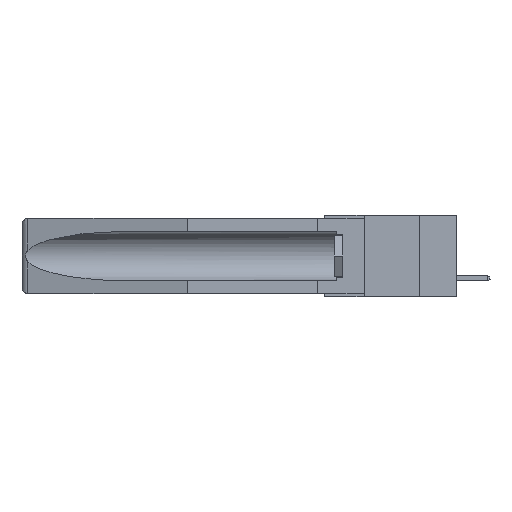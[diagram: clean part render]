
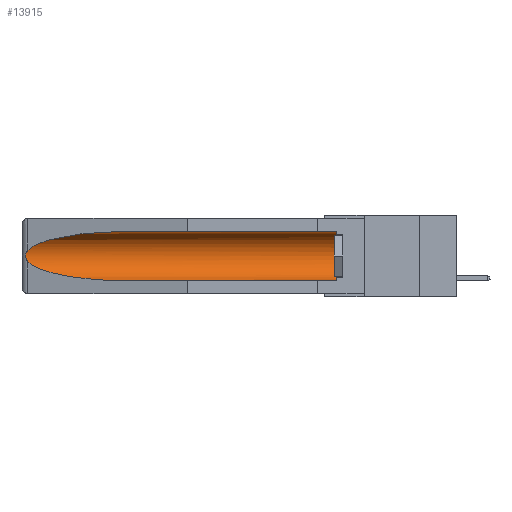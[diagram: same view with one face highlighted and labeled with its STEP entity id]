
A CAD part, left-side view. The second image highlights one B-rep face of the part: STEP entity #13915.
In plain terms, the highlighted cylindrical face has radius 2.857 mm (diameter 5.715 mm), a partial arc.
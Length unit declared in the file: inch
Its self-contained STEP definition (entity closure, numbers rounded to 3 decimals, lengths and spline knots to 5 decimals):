
#265 = EDGE_CURVE ( 'NONE', #20814, #21322, #21189, .T. ) ;
#880 = VERTEX_POINT ( 'NONE', #18249 ) ;
#1745 = CARTESIAN_POINT ( 'NONE',  ( 0.155, 0.126, -0.059 ) ) ;
#2369 = EDGE_CURVE ( 'NONE', #880, #20814, #8147, .T. ) ;
#2906 = CARTESIAN_POINT ( 'NONE',  ( 0.2675, 1.53308, -0.16763 ) ) ;
#2974 = CARTESIAN_POINT ( 'NONE',  ( 0.2673, 1.53269, -0.17917 ) ) ;
#3611 =( BOUNDED_CURVE ( )  B_SPLINE_CURVE ( 3, ( #19361, #7776, #17625, #17774 ),
 .UNSPECIFIED., .F., .F. ) 
 B_SPLINE_CURVE_WITH_KNOTS ( ( 4, 4 ),
 ( 0.1948, 1.5708 ),
 .UNSPECIFIED. ) 
 CURVE ( )  GEOMETRIC_REPRESENTATION_ITEM ( )  RATIONAL_B_SPLINE_CURVE ( ( 1., 0.848, 0.848, 1. ) ) 
 REPRESENTATION_ITEM ( '' )  );
#3753 = VERTEX_POINT ( 'NONE', #19304 ) ;
#3755 = CARTESIAN_POINT ( 'NONE',  ( 0.155, -0.30754, -0.1715 ) ) ;
#3777 = CARTESIAN_POINT ( 'NONE',  ( 0.155, 1.07973, -0.059 ) ) ;
#5755 = VERTEX_POINT ( 'NONE', #14156 ) ;
#6045 = CARTESIAN_POINT ( 'NONE',  ( 0.26537, 1.52718, -0.14972 ) ) ;
#6341 = CARTESIAN_POINT ( 'NONE',  ( 0.2675, 1.53308, -0.17534 ) ) ;
#6911 = CARTESIAN_POINT ( 'NONE',  ( 0.155, -0.30754, -0.284 ) ) ;
#7776 = CARTESIAN_POINT ( 'NONE',  ( 0.25451, 1.48313, -0.24835 ) ) ;
#7859 = CARTESIAN_POINT ( 'NONE',  ( 0.26537, 1.52718, -0.14972 ) ) ;
#7913 = DIRECTION ( 'NONE',  ( 0., 1., 0. ) ) ;
#8147 = CIRCLE ( 'NONE', #18704, 0.1125 ) ;
#9246 = CYLINDRICAL_SURFACE ( 'NONE', #20652, 0.1125 ) ;
#9306 = EDGE_CURVE ( 'NONE', #3753, #20922, #3611, .T. ) ;
#9915 = EDGE_CURVE ( 'NONE', #21322, #5755, #17525, .T. ) ;
#11188 = CARTESIAN_POINT ( 'NONE',  ( 0.2673, 1.5327, -0.16383 ) ) ;
#11540 = CARTESIAN_POINT ( 'NONE',  ( 0.155, 1.07973, -0.059 ) ) ;
#11733 = ORIENTED_EDGE ( 'NONE', *, *, #2369, .T. ) ;
#11760 = ORIENTED_EDGE ( 'NONE', *, *, #9306, .T. ) ;
#11868 = DIRECTION ( 'NONE',  ( 0., -1., 0. ) ) ;
#11953 = EDGE_CURVE ( 'NONE', #880, #20922, #21327, .T. ) ;
#12131 = DIRECTION ( 'NONE',  ( 0., 0., 1. ) ) ;
#12269 = CARTESIAN_POINT ( 'NONE',  ( 0.155, 1.07973, -0.284 ) ) ;
#12588 = CARTESIAN_POINT ( 'NONE',  ( 0.25451, 1.48313, -0.09465 ) ) ;
#12850 = ORIENTED_EDGE ( 'NONE', *, *, #265, .T. ) ;
#13094 = EDGE_CURVE ( 'NONE', #5755, #3753, #15914, .T. ) ;
#13401 = DIRECTION ( 'NONE',  ( 0., 1., 0. ) ) ;
#13672 = ORIENTED_EDGE ( 'NONE', *, *, #9915, .T. ) ;
#13698 = VECTOR ( 'NONE', #7913, 39.37008 ) ;
#13915 = ADVANCED_FACE ( 'NONE', ( #18108 ), #9246, .F. ) ;
#14126 = ORIENTED_EDGE ( 'NONE', *, *, #13094, .T. ) ;
#14156 = CARTESIAN_POINT ( 'NONE',  ( 0.26537, 1.52718, -0.14972 ) ) ;
#14692 = CARTESIAN_POINT ( 'NONE',  ( 0.155, -0.30754, -0.059 ) ) ;
#15372 = CARTESIAN_POINT ( 'NONE',  ( 0.155, 0.126, -0.1715 ) ) ;
#15914 = B_SPLINE_CURVE_WITH_KNOTS ( 'NONE', 3,
 ( #7859, #17640, #21138, #11188, #2906, #6341, #2974, #16301, #17924, #17995 ),
 .UNSPECIFIED., .F., .F.,
 ( 4, 2, 2, 2, 4 ),
 ( 0., 0.00029, 0.00058, 0.00087, 0.00117 ),
 .UNSPECIFIED. ) ;
#16301 = CARTESIAN_POINT ( 'NONE',  ( 0.26655, 1.53094, -0.18657 ) ) ;
#16480 = ORIENTED_EDGE ( 'NONE', *, *, #11953, .F. ) ;
#16670 = VECTOR ( 'NONE', #13401, 39.37008 ) ;
#17525 =( BOUNDED_CURVE ( )  B_SPLINE_CURVE ( 3, ( #3777, #17557, #12588, #6045 ),
 .UNSPECIFIED., .F., .F. ) 
 B_SPLINE_CURVE_WITH_KNOTS ( ( 4, 4 ),
 ( 4.71239, 6.08839 ),
 .UNSPECIFIED. ) 
 CURVE ( )  GEOMETRIC_REPRESENTATION_ITEM ( )  RATIONAL_B_SPLINE_CURVE ( ( 1., 0.848, 0.848, 1. ) ) 
 REPRESENTATION_ITEM ( '' )  );
#17557 = CARTESIAN_POINT ( 'NONE',  ( 0.21114, 1.30732, -0.059 ) ) ;
#17625 = CARTESIAN_POINT ( 'NONE',  ( 0.21114, 1.30732, -0.284 ) ) ;
#17640 = CARTESIAN_POINT ( 'NONE',  ( 0.26597, 1.52961, -0.15275 ) ) ;
#17774 = CARTESIAN_POINT ( 'NONE',  ( 0.155, 1.07973, -0.284 ) ) ;
#17800 = EDGE_LOOP ( 'NONE', ( #13672, #14126, #11760, #16480, #11733, #12850 ) ) ;
#17924 = CARTESIAN_POINT ( 'NONE',  ( 0.26597, 1.5296, -0.19026 ) ) ;
#17995 = CARTESIAN_POINT ( 'NONE',  ( 0.26537, 1.52718, -0.19328 ) ) ;
#18108 = FACE_OUTER_BOUND ( 'NONE', #17800, .T. ) ;
#18249 = CARTESIAN_POINT ( 'NONE',  ( 0.155, 0.126, -0.284 ) ) ;
#18361 = DIRECTION ( 'NONE',  ( 0., 0., 1. ) ) ;
#18704 = AXIS2_PLACEMENT_3D ( 'NONE', #15372, #11868, #18361 ) ;
#19304 = CARTESIAN_POINT ( 'NONE',  ( 0.26537, 1.52718, -0.19328 ) ) ;
#19361 = CARTESIAN_POINT ( 'NONE',  ( 0.26537, 1.52718, -0.19328 ) ) ;
#20652 = AXIS2_PLACEMENT_3D ( 'NONE', #3755, #20679, #12131 ) ;
#20679 = DIRECTION ( 'NONE',  ( 0., 1., 0. ) ) ;
#20814 = VERTEX_POINT ( 'NONE', #1745 ) ;
#20922 = VERTEX_POINT ( 'NONE', #12269 ) ;
#21138 = CARTESIAN_POINT ( 'NONE',  ( 0.26654, 1.53092, -0.15636 ) ) ;
#21189 = LINE ( 'NONE', #14692, #13698 ) ;
#21322 = VERTEX_POINT ( 'NONE', #11540 ) ;
#21327 = LINE ( 'NONE', #6911, #16670 ) ;
